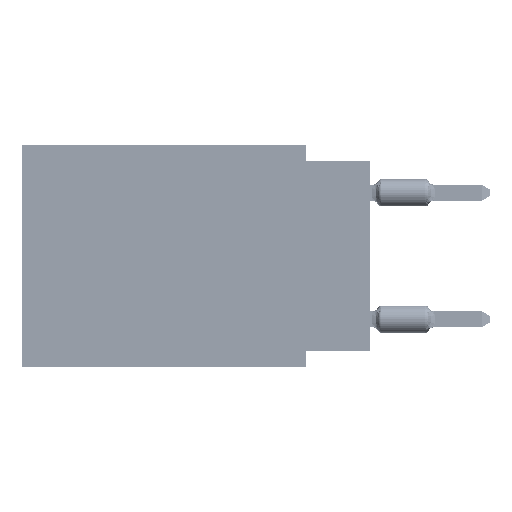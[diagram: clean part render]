
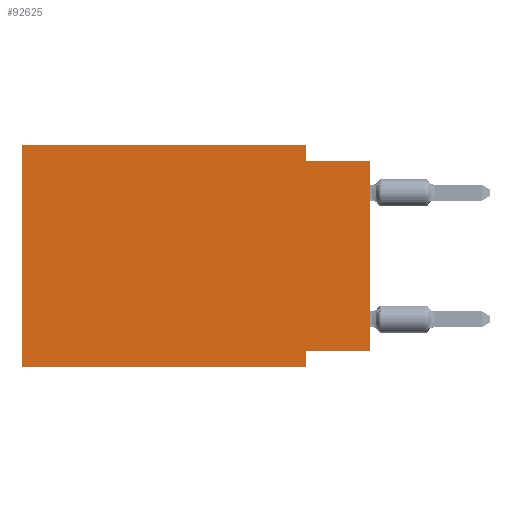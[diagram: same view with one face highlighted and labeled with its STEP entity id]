
A CAD part, left-side view. The second image highlights one B-rep face of the part: STEP entity #92625.
In plain terms, the highlighted planar face has unit normal (-1, 0, 0).
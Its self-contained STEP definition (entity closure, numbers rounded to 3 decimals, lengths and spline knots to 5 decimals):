
#2028 = ORIENTED_EDGE ( 'NONE', *, *, #117687, .F. ) ;
#2204 = ORIENTED_EDGE ( 'NONE', *, *, #29288, .F. ) ;
#2254 = CARTESIAN_POINT ( 'NONE',  ( 0., 0., 0. ) ) ;
#3498 = DIRECTION ( 'NONE',  ( 0., -1., 0. ) ) ;
#4131 = CARTESIAN_POINT ( 'NONE',  ( 0., 0.55, 0. ) ) ;
#10334 = VERTEX_POINT ( 'NONE', #63638 ) ;
#11911 = DIRECTION ( 'NONE',  ( 0., 1., 0. ) ) ;
#13484 = DIRECTION ( 'NONE',  ( 0., -1., 0. ) ) ;
#14064 = CARTESIAN_POINT ( 'NONE',  ( 0., 0., -0.325 ) ) ;
#16288 = VERTEX_POINT ( 'NONE', #14064 ) ;
#19543 = LINE ( 'NONE', #93130, #56219 ) ;
#19817 = CARTESIAN_POINT ( 'NONE',  ( 0., 0., -0.325 ) ) ;
#19892 = EDGE_CURVE ( 'NONE', #70191, #118249, #106248, .T. ) ;
#20416 = LINE ( 'NONE', #19817, #64765 ) ;
#22961 = DIRECTION ( 'NONE',  ( 0., -1., 0. ) ) ;
#23024 = EDGE_CURVE ( 'NONE', #16288, #97941, #94066, .T. ) ;
#29288 = EDGE_CURVE ( 'NONE', #63239, #10334, #51908, .T. ) ;
#30914 = DIRECTION ( 'NONE',  ( 0., 0., -1. ) ) ;
#32326 = LINE ( 'NONE', #32924, #57952 ) ;
#32924 = CARTESIAN_POINT ( 'NONE',  ( 0., 0.55, -0.35 ) ) ;
#34130 = CARTESIAN_POINT ( 'NONE',  ( 0., 0.1, 0. ) ) ;
#35203 = VECTOR ( 'NONE', #3498, 39.37008 ) ;
#37741 = ORIENTED_EDGE ( 'NONE', *, *, #19892, .F. ) ;
#37966 = VECTOR ( 'NONE', #22961, 39.37008 ) ;
#42375 = ORIENTED_EDGE ( 'NONE', *, *, #68371, .T. ) ;
#44581 = CARTESIAN_POINT ( 'NONE',  ( 0., 0.1, -0.35 ) ) ;
#47881 = DIRECTION ( 'NONE',  ( 0., 0., 1. ) ) ;
#48974 = VECTOR ( 'NONE', #116334, 39.37008 ) ;
#51908 = LINE ( 'NONE', #44581, #48974 ) ;
#52149 = CARTESIAN_POINT ( 'NONE',  ( 0., 0.1, -0.025 ) ) ;
#56219 = VECTOR ( 'NONE', #57252, 39.37008 ) ;
#56952 = VERTEX_POINT ( 'NONE', #110309 ) ;
#57252 = DIRECTION ( 'NONE',  ( 0., 0., -1. ) ) ;
#57445 = CARTESIAN_POINT ( 'NONE',  ( 0., 0.55, 0. ) ) ;
#57952 = VECTOR ( 'NONE', #13484, 39.37008 ) ;
#63239 = VERTEX_POINT ( 'NONE', #94312 ) ;
#63638 = CARTESIAN_POINT ( 'NONE',  ( 0., 0.1, -0.35 ) ) ;
#64765 = VECTOR ( 'NONE', #11911, 39.37008 ) ;
#67510 = EDGE_LOOP ( 'NONE', ( #68310, #69653, #70888, #37741, #2028, #42375, #2204, #93449 ) ) ;
#68310 = ORIENTED_EDGE ( 'NONE', *, *, #23024, .T. ) ;
#68369 = LINE ( 'NONE', #57445, #72222 ) ;
#68371 = EDGE_CURVE ( 'NONE', #56952, #10334, #32326, .T. ) ;
#69653 = ORIENTED_EDGE ( 'NONE', *, *, #97188, .F. ) ;
#69781 = EDGE_CURVE ( 'NONE', #118249, #85500, #19543, .T. ) ;
#70191 = VERTEX_POINT ( 'NONE', #97917 ) ;
#70888 = ORIENTED_EDGE ( 'NONE', *, *, #69781, .F. ) ;
#72222 = VECTOR ( 'NONE', #96313, 39.37008 ) ;
#77110 = VECTOR ( 'NONE', #47881, 39.37008 ) ;
#77683 = LINE ( 'NONE', #86783, #35203 ) ;
#84598 = EDGE_CURVE ( 'NONE', #16288, #63239, #20416, .T. ) ;
#85500 = VERTEX_POINT ( 'NONE', #52149 ) ;
#86783 = CARTESIAN_POINT ( 'NONE',  ( 0., 0., -0.025 ) ) ;
#87435 = FACE_OUTER_BOUND ( 'NONE', #67510, .T. ) ;
#92625 = ADVANCED_FACE ( 'NONE', ( #87435 ), #114191, .F. ) ;
#93130 = CARTESIAN_POINT ( 'NONE',  ( 0., 0.1, 0. ) ) ;
#93449 = ORIENTED_EDGE ( 'NONE', *, *, #84598, .F. ) ;
#94066 = LINE ( 'NONE', #2254, #77110 ) ;
#94312 = CARTESIAN_POINT ( 'NONE',  ( 0., 0.1, -0.325 ) ) ;
#96313 = DIRECTION ( 'NONE',  ( 0., 0., 1. ) ) ;
#97188 = EDGE_CURVE ( 'NONE', #85500, #97941, #77683, .T. ) ;
#97917 = CARTESIAN_POINT ( 'NONE',  ( 0., 0.55, 0. ) ) ;
#97941 = VERTEX_POINT ( 'NONE', #102933 ) ;
#102933 = CARTESIAN_POINT ( 'NONE',  ( 0., 0., -0.025 ) ) ;
#105029 = CARTESIAN_POINT ( 'NONE',  ( 0., 0.55, 0. ) ) ;
#106248 = LINE ( 'NONE', #105029, #37966 ) ;
#110309 = CARTESIAN_POINT ( 'NONE',  ( 0., 0.55, -0.35 ) ) ;
#112344 = AXIS2_PLACEMENT_3D ( 'NONE', #4131, #112371, #30914 ) ;
#112371 = DIRECTION ( 'NONE',  ( 1., 0., 0. ) ) ;
#114191 = PLANE ( 'NONE',  #112344 ) ;
#116334 = DIRECTION ( 'NONE',  ( 0., 0., -1. ) ) ;
#117687 = EDGE_CURVE ( 'NONE', #56952, #70191, #68369, .T. ) ;
#118249 = VERTEX_POINT ( 'NONE', #34130 ) ;
